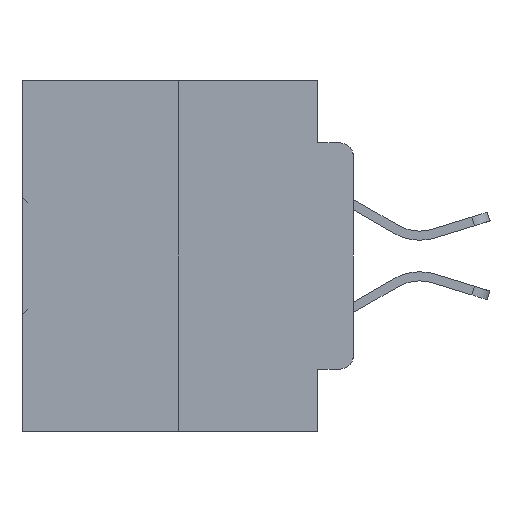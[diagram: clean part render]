
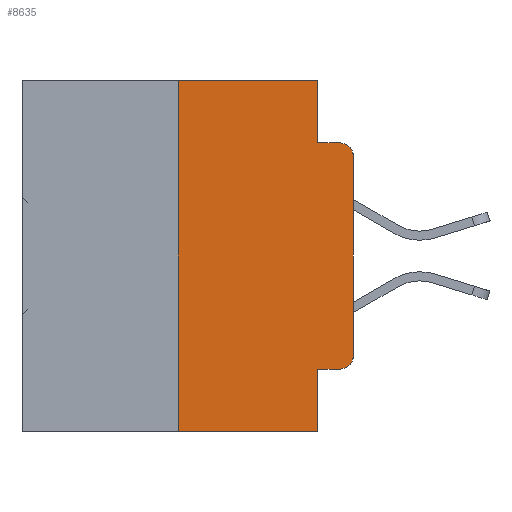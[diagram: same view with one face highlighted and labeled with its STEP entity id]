
A CAD part, left-side view. The second image highlights one B-rep face of the part: STEP entity #8635.
In plain terms, the highlighted planar face has unit normal (-1, 0, 0).
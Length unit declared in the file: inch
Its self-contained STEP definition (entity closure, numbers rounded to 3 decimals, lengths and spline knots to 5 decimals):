
#54 = LINE ( 'NONE', #21788, #13785 ) ;
#500 = CARTESIAN_POINT ( 'NONE',  ( 0., 0.02, -0.1085 ) ) ;
#669 = ORIENTED_EDGE ( 'NONE', *, *, #23239, .F. ) ;
#1254 = EDGE_CURVE ( 'NONE', #19545, #3001, #28581, .T. ) ;
#1383 = ORIENTED_EDGE ( 'NONE', *, *, #28593, .F. ) ;
#1476 = ORIENTED_EDGE ( 'NONE', *, *, #11835, .F. ) ;
#2574 = CARTESIAN_POINT ( 'NONE',  ( 0., 0.051, 0. ) ) ;
#2608 = EDGE_CURVE ( 'NONE', #10692, #30260, #34628, .T. ) ;
#3001 = VERTEX_POINT ( 'NONE', #21718 ) ;
#3126 = ORIENTED_EDGE ( 'NONE', *, *, #1254, .T. ) ;
#3288 = DIRECTION ( 'NONE',  ( 0., 0., -1. ) ) ;
#3337 = CARTESIAN_POINT ( 'NONE',  ( 0., 0.25, 0. ) ) ;
#3654 = VERTEX_POINT ( 'NONE', #3337 ) ;
#3812 = VECTOR ( 'NONE', #19350, 39.37008 ) ;
#4393 = ORIENTED_EDGE ( 'NONE', *, *, #14342, .F. ) ;
#4507 = LINE ( 'NONE', #19711, #24282 ) ;
#4734 = ORIENTED_EDGE ( 'NONE', *, *, #25652, .T. ) ;
#5171 = DIRECTION ( 'NONE',  ( 0., 0., -1. ) ) ;
#5595 = VERTEX_POINT ( 'NONE', #9851 ) ;
#5617 = DIRECTION ( 'NONE',  ( 0., -1., 0. ) ) ;
#5736 = ORIENTED_EDGE ( 'NONE', *, *, #26096, .T. ) ;
#6151 = AXIS2_PLACEMENT_3D ( 'NONE', #16219, #34629, #18923 ) ;
#6162 = ORIENTED_EDGE ( 'NONE', *, *, #11135, .T. ) ;
#6406 = VECTOR ( 'NONE', #11764, 39.37008 ) ;
#6507 = CARTESIAN_POINT ( 'NONE',  ( 0., 0.051, -0.4115 ) ) ;
#8635 = ADVANCED_FACE ( 'NONE', ( #12029 ), #34437, .F. ) ;
#9040 = CARTESIAN_POINT ( 'NONE',  ( 0., 0.051, 0. ) ) ;
#9706 = CARTESIAN_POINT ( 'NONE',  ( 0., 0., -0.3915 ) ) ;
#9851 = CARTESIAN_POINT ( 'NONE',  ( 0., 0., -0.1085 ) ) ;
#10063 = DIRECTION ( 'NONE',  ( 0., -1., 0. ) ) ;
#10692 = VERTEX_POINT ( 'NONE', #13847 ) ;
#10928 = CARTESIAN_POINT ( 'NONE',  ( 0., 0., 0. ) ) ;
#11077 = LINE ( 'NONE', #16648, #3812 ) ;
#11111 = CARTESIAN_POINT ( 'NONE',  ( 0., 0.473, -0.5 ) ) ;
#11135 = EDGE_CURVE ( 'NONE', #26513, #17853, #23123, .T. ) ;
#11764 = DIRECTION ( 'NONE',  ( 0., -1., 0. ) ) ;
#11835 = EDGE_CURVE ( 'NONE', #19545, #3654, #4507, .T. ) ;
#12029 = FACE_OUTER_BOUND ( 'NONE', #12150, .T. ) ;
#12150 = EDGE_LOOP ( 'NONE', ( #4734, #20033, #28640, #669, #1383, #1476, #3126, #4393, #5736, #6162 ) ) ;
#13785 = VECTOR ( 'NONE', #5617, 39.37008 ) ;
#13847 = CARTESIAN_POINT ( 'NONE',  ( 0., 0.051, -0.0885 ) ) ;
#14342 = EDGE_CURVE ( 'NONE', #34736, #3001, #34689, .T. ) ;
#14405 = DIRECTION ( 'NONE',  ( 0., 0., -1. ) ) ;
#14489 = VECTOR ( 'NONE', #14405, 39.37008 ) ;
#16219 = CARTESIAN_POINT ( 'NONE',  ( 0., 0.02, -0.3915 ) ) ;
#16648 = CARTESIAN_POINT ( 'NONE',  ( 0., 0.051, 0. ) ) ;
#17853 = VERTEX_POINT ( 'NONE', #9706 ) ;
#18734 = CARTESIAN_POINT ( 'NONE',  ( 0., 0.473, 0. ) ) ;
#18923 = DIRECTION ( 'NONE',  ( 0., 0., -1. ) ) ;
#19350 = DIRECTION ( 'NONE',  ( 0., 0., -1. ) ) ;
#19545 = VERTEX_POINT ( 'NONE', #29854 ) ;
#19591 = DIRECTION ( 'NONE',  ( -1., 0., 0. ) ) ;
#19711 = CARTESIAN_POINT ( 'NONE',  ( 0., 0.25, 0. ) ) ;
#19841 = LINE ( 'NONE', #10928, #25980 ) ;
#19953 = VERTEX_POINT ( 'NONE', #2574 ) ;
#20033 = ORIENTED_EDGE ( 'NONE', *, *, #27387, .T. ) ;
#21259 = AXIS2_PLACEMENT_3D ( 'NONE', #18734, #21372, #5171 ) ;
#21372 = DIRECTION ( 'NONE',  ( 1., 0., 0. ) ) ;
#21495 = VECTOR ( 'NONE', #27629, 39.37008 ) ;
#21511 = VECTOR ( 'NONE', #10063, 39.37008 ) ;
#21718 = CARTESIAN_POINT ( 'NONE',  ( 0., 0.051, -0.5 ) ) ;
#21788 = CARTESIAN_POINT ( 'NONE',  ( 0., 0.473, 0. ) ) ;
#22330 = LINE ( 'NONE', #25943, #21511 ) ;
#23123 = CIRCLE ( 'NONE', #6151, 0.02 ) ;
#23239 = EDGE_CURVE ( 'NONE', #19953, #10692, #11077, .T. ) ;
#24282 = VECTOR ( 'NONE', #32808, 39.37008 ) ;
#25652 = EDGE_CURVE ( 'NONE', #17853, #5595, #19841, .T. ) ;
#25943 = CARTESIAN_POINT ( 'NONE',  ( 0., 0.051, -0.4115 ) ) ;
#25980 = VECTOR ( 'NONE', #26876, 39.37008 ) ;
#26096 = EDGE_CURVE ( 'NONE', #34736, #26513, #22330, .T. ) ;
#26513 = VERTEX_POINT ( 'NONE', #34200 ) ;
#26647 = CARTESIAN_POINT ( 'NONE',  ( 0., 0.051, -0.0885 ) ) ;
#26876 = DIRECTION ( 'NONE',  ( 0., 0., 1. ) ) ;
#27387 = EDGE_CURVE ( 'NONE', #5595, #30260, #32531, .T. ) ;
#27629 = DIRECTION ( 'NONE',  ( 0., -1., 0. ) ) ;
#28581 = LINE ( 'NONE', #11111, #6406 ) ;
#28593 = EDGE_CURVE ( 'NONE', #3654, #19953, #54, .T. ) ;
#28640 = ORIENTED_EDGE ( 'NONE', *, *, #2608, .F. ) ;
#29854 = CARTESIAN_POINT ( 'NONE',  ( 0., 0.25, -0.5 ) ) ;
#30260 = VERTEX_POINT ( 'NONE', #30956 ) ;
#30956 = CARTESIAN_POINT ( 'NONE',  ( 0., 0.02, -0.0885 ) ) ;
#32531 = CIRCLE ( 'NONE', #33347, 0.02 ) ;
#32808 = DIRECTION ( 'NONE',  ( 0., 0., 1. ) ) ;
#33347 = AXIS2_PLACEMENT_3D ( 'NONE', #500, #19591, #3288 ) ;
#34200 = CARTESIAN_POINT ( 'NONE',  ( 0., 0.02, -0.4115 ) ) ;
#34437 = PLANE ( 'NONE',  #21259 ) ;
#34628 = LINE ( 'NONE', #26647, #21495 ) ;
#34629 = DIRECTION ( 'NONE',  ( -1., 0., 0. ) ) ;
#34689 = LINE ( 'NONE', #9040, #14489 ) ;
#34736 = VERTEX_POINT ( 'NONE', #6507 ) ;
